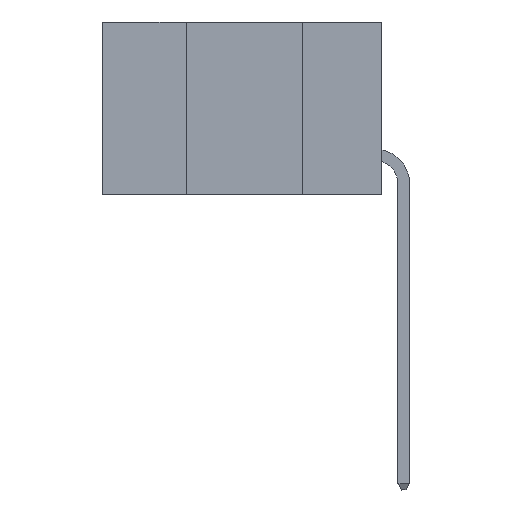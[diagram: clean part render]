
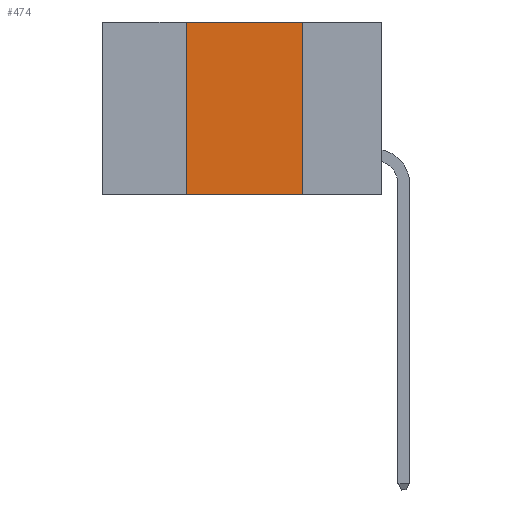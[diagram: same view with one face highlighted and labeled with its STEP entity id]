
A CAD part, left-side view. The second image highlights one B-rep face of the part: STEP entity #474.
In plain terms, the highlighted planar face has unit normal (-1, 0, 0).
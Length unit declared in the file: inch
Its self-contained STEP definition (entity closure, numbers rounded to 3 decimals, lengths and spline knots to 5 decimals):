
#474 = ADVANCED_FACE ( 'NONE', ( #29809 ), #3665, .F. ) ;
#1895 = DIRECTION ( 'NONE',  ( 0., 0., 1. ) ) ;
#3665 = PLANE ( 'NONE',  #26288 ) ;
#4297 = CARTESIAN_POINT ( 'NONE',  ( 0., 0.17, 0. ) ) ;
#5087 = CARTESIAN_POINT ( 'NONE',  ( 0., 0.42, 0. ) ) ;
#6088 = CARTESIAN_POINT ( 'NONE',  ( 0., 0.17, 0. ) ) ;
#8311 = VERTEX_POINT ( 'NONE', #47300 ) ;
#8647 = EDGE_CURVE ( 'NONE', #38690, #41291, #22579, .T. ) ;
#8824 = DIRECTION ( 'NONE',  ( 1., 0., 0. ) ) ;
#9016 = CARTESIAN_POINT ( 'NONE',  ( 0., 0.6, 0. ) ) ;
#9211 = DIRECTION ( 'NONE',  ( 0., 0., -1. ) ) ;
#11370 = ORIENTED_EDGE ( 'NONE', *, *, #31107, .F. ) ;
#14808 = LINE ( 'NONE', #34756, #41895 ) ;
#16168 = DIRECTION ( 'NONE',  ( 0., 0., -1. ) ) ;
#16348 = ORIENTED_EDGE ( 'NONE', *, *, #16896, .T. ) ;
#16492 = VECTOR ( 'NONE', #1895, 39.37008 ) ;
#16896 = EDGE_CURVE ( 'NONE', #8311, #40907, #14808, .T. ) ;
#19127 = LINE ( 'NONE', #4297, #24527 ) ;
#22579 = LINE ( 'NONE', #26273, #41828 ) ;
#23146 = CARTESIAN_POINT ( 'NONE',  ( 0., 0.17, -0.37 ) ) ;
#24034 = EDGE_LOOP ( 'NONE', ( #11370, #29899, #30968, #16348 ) ) ;
#24527 = VECTOR ( 'NONE', #9211, 39.37008 ) ;
#26273 = CARTESIAN_POINT ( 'NONE',  ( 0., 0.6, 0. ) ) ;
#26288 = AXIS2_PLACEMENT_3D ( 'NONE', #9016, #8824, #16168 ) ;
#26442 = DIRECTION ( 'NONE',  ( 0., -1., 0. ) ) ;
#29809 = FACE_OUTER_BOUND ( 'NONE', #24034, .T. ) ;
#29899 = ORIENTED_EDGE ( 'NONE', *, *, #8647, .F. ) ;
#30400 = DIRECTION ( 'NONE',  ( 0., -1., 0. ) ) ;
#30968 = ORIENTED_EDGE ( 'NONE', *, *, #31815, .F. ) ;
#31107 = EDGE_CURVE ( 'NONE', #41291, #40907, #19127, .T. ) ;
#31815 = EDGE_CURVE ( 'NONE', #8311, #38690, #42307, .T. ) ;
#34756 = CARTESIAN_POINT ( 'NONE',  ( 0., 0.6, -0.37 ) ) ;
#38690 = VERTEX_POINT ( 'NONE', #48922 ) ;
#40907 = VERTEX_POINT ( 'NONE', #23146 ) ;
#41291 = VERTEX_POINT ( 'NONE', #6088 ) ;
#41828 = VECTOR ( 'NONE', #26442, 39.37008 ) ;
#41895 = VECTOR ( 'NONE', #30400, 39.37008 ) ;
#42307 = LINE ( 'NONE', #5087, #16492 ) ;
#47300 = CARTESIAN_POINT ( 'NONE',  ( 0., 0.42, -0.37 ) ) ;
#48922 = CARTESIAN_POINT ( 'NONE',  ( 0., 0.42, 0. ) ) ;
